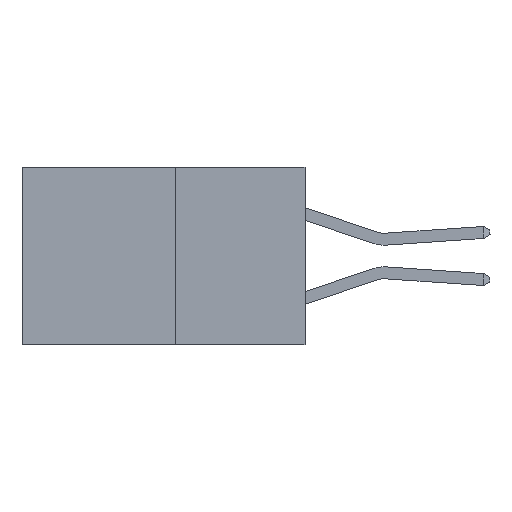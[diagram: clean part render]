
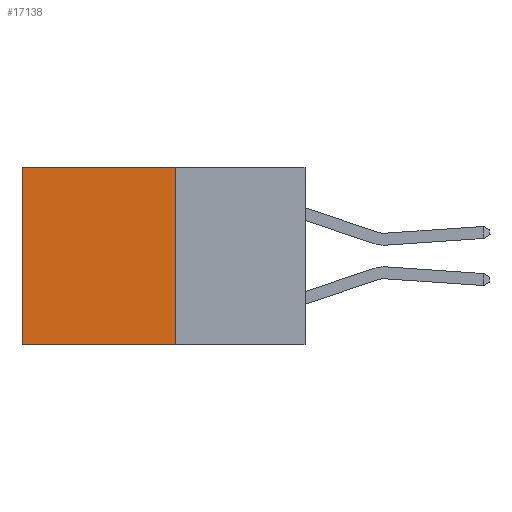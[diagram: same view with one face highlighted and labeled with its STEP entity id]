
A CAD part, left-side view. The second image highlights one B-rep face of the part: STEP entity #17138.
In plain terms, the highlighted planar face has unit normal (-1, 0, 0).
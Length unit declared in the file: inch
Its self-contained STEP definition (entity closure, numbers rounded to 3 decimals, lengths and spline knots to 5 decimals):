
#124 = CARTESIAN_POINT ( 'NONE',  ( 0.277, 0.59, -0.37 ) ) ;
#214 = LINE ( 'NONE', #1701, #3930 ) ;
#245 = EDGE_CURVE ( 'NONE', #6856, #2218, #19740, .T. ) ;
#1377 = EDGE_LOOP ( 'NONE', ( #5261, #17173, #13804, #13076 ) ) ;
#1701 = CARTESIAN_POINT ( 'NONE',  ( 0.277, 0.27, 0. ) ) ;
#1771 = DIRECTION ( 'NONE',  ( 0., 1., 0. ) ) ;
#2218 = VERTEX_POINT ( 'NONE', #18612 ) ;
#3335 = LINE ( 'NONE', #16599, #15553 ) ;
#3459 = CARTESIAN_POINT ( 'NONE',  ( 0.277, 0.27, 0. ) ) ;
#3930 = VECTOR ( 'NONE', #1771, 39.37008 ) ;
#5261 = ORIENTED_EDGE ( 'NONE', *, *, #5999, .T. ) ;
#5999 = EDGE_CURVE ( 'NONE', #18113, #16028, #10682, .T. ) ;
#6415 = PLANE ( 'NONE',  #10309 ) ;
#6840 = VECTOR ( 'NONE', #20313, 39.37008 ) ;
#6856 = VERTEX_POINT ( 'NONE', #3459 ) ;
#7315 = VECTOR ( 'NONE', #10667, 39.37008 ) ;
#8086 = DIRECTION ( 'NONE',  ( 0., 0., -1. ) ) ;
#9832 = EDGE_CURVE ( 'NONE', #6856, #18113, #214, .T. ) ;
#10263 = CARTESIAN_POINT ( 'NONE',  ( 0.277, 0.27, -0.37 ) ) ;
#10309 = AXIS2_PLACEMENT_3D ( 'NONE', #15914, #17466, #8086 ) ;
#10667 = DIRECTION ( 'NONE',  ( 0., 0., -1. ) ) ;
#10682 = LINE ( 'NONE', #15080, #6840 ) ;
#11979 = CARTESIAN_POINT ( 'NONE',  ( 0.277, 0.59, 0. ) ) ;
#13076 = ORIENTED_EDGE ( 'NONE', *, *, #9832, .T. ) ;
#13494 = DIRECTION ( 'NONE',  ( 0., 1., 0. ) ) ;
#13804 = ORIENTED_EDGE ( 'NONE', *, *, #245, .F. ) ;
#15080 = CARTESIAN_POINT ( 'NONE',  ( 0.277, 0.59, -0.37 ) ) ;
#15553 = VECTOR ( 'NONE', #13494, 39.37008 ) ;
#15914 = CARTESIAN_POINT ( 'NONE',  ( 0.277, 0.27, -0.37 ) ) ;
#16028 = VERTEX_POINT ( 'NONE', #124 ) ;
#16599 = CARTESIAN_POINT ( 'NONE',  ( 0.277, 0.27, -0.37 ) ) ;
#16763 = FACE_OUTER_BOUND ( 'NONE', #1377, .T. ) ;
#16978 = EDGE_CURVE ( 'NONE', #2218, #16028, #3335, .T. ) ;
#17138 = ADVANCED_FACE ( 'NONE', ( #16763 ), #6415, .F. ) ;
#17173 = ORIENTED_EDGE ( 'NONE', *, *, #16978, .F. ) ;
#17466 = DIRECTION ( 'NONE',  ( 1., 0., 0. ) ) ;
#18113 = VERTEX_POINT ( 'NONE', #11979 ) ;
#18612 = CARTESIAN_POINT ( 'NONE',  ( 0.277, 0.27, -0.37 ) ) ;
#19740 = LINE ( 'NONE', #10263, #7315 ) ;
#20313 = DIRECTION ( 'NONE',  ( 0., 0., -1. ) ) ;
